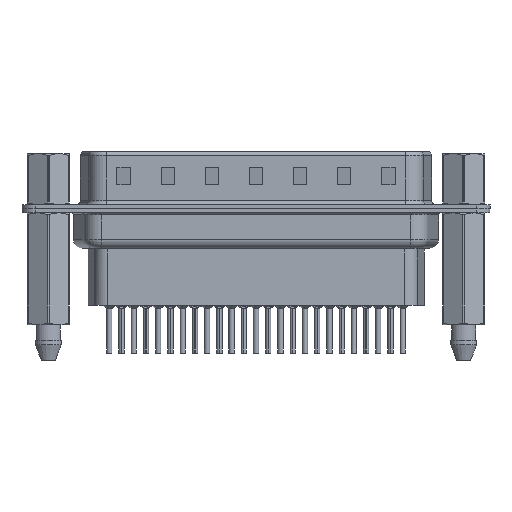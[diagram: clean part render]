
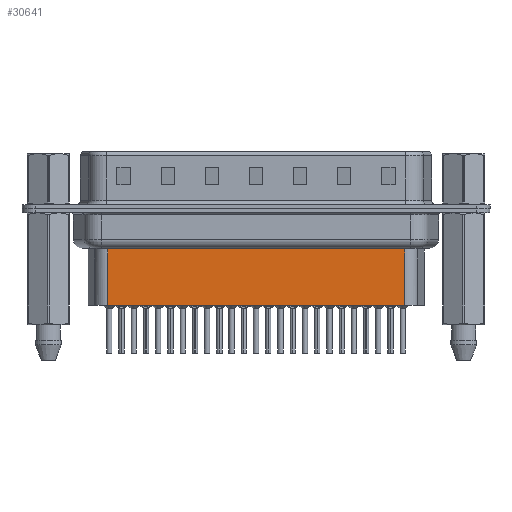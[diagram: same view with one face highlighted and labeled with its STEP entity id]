
A CAD part, front view. The second image highlights one B-rep face of the part: STEP entity #30641.
In plain terms, the highlighted planar face has unit normal (0, -1, 0).
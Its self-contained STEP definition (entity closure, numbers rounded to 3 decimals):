
#833 = AXIS2_PLACEMENT_3D ( 'NONE', #12504, #2280, #27858 ) ;
#1153 = ORIENTED_EDGE ( 'NONE', *, *, #26784, .F. ) ;
#1212 = EDGE_CURVE ( 'NONE', #7020, #14730, #2708, .T. ) ;
#2215 = EDGE_CURVE ( 'NONE', #14730, #2582, #17386, .T. ) ;
#2280 = DIRECTION ( 'NONE',  ( 0., -1., 0. ) ) ;
#2431 = PLANE ( 'NONE',  #833 ) ;
#2582 = VERTEX_POINT ( 'NONE', #17031 ) ;
#2708 = LINE ( 'NONE', #30763, #29126 ) ;
#4353 = VERTEX_POINT ( 'NONE', #31399 ) ;
#6843 = LINE ( 'NONE', #19389, #10309 ) ;
#7020 = VERTEX_POINT ( 'NONE', #22958 ) ;
#7847 = CARTESIAN_POINT ( 'NONE',  ( 40.344, -3.5, -3.1 ) ) ;
#10309 = VECTOR ( 'NONE', #21712, 1000. ) ;
#12504 = CARTESIAN_POINT ( 'NONE',  ( 6.706, -3.5, -3.1 ) ) ;
#13961 = ORIENTED_EDGE ( 'NONE', *, *, #1212, .T. ) ;
#14730 = VERTEX_POINT ( 'NONE', #31713 ) ;
#15062 = DIRECTION ( 'NONE',  ( 0., 0., -1. ) ) ;
#15328 = FACE_OUTER_BOUND ( 'NONE', #32353, .T. ) ;
#17031 = CARTESIAN_POINT ( 'NONE',  ( 6.706, -3.5, -10.95 ) ) ;
#17386 = LINE ( 'NONE', #27608, #23656 ) ;
#17885 = ORIENTED_EDGE ( 'NONE', *, *, #2215, .T. ) ;
#19389 = CARTESIAN_POINT ( 'NONE',  ( 6.706, -3.5, -10.95 ) ) ;
#20243 = LINE ( 'NONE', #7847, #20728 ) ;
#20728 = VECTOR ( 'NONE', #27650, 1000. ) ;
#21712 = DIRECTION ( 'NONE',  ( -1., 0., 0. ) ) ;
#22958 = CARTESIAN_POINT ( 'NONE',  ( 40.344, -3.5, -4.097 ) ) ;
#23656 = VECTOR ( 'NONE', #15062, 1000. ) ;
#24851 = ORIENTED_EDGE ( 'NONE', *, *, #28552, .F. ) ;
#26784 = EDGE_CURVE ( 'NONE', #7020, #4353, #20243, .T. ) ;
#27608 = CARTESIAN_POINT ( 'NONE',  ( 6.706, -3.5, -3.1 ) ) ;
#27650 = DIRECTION ( 'NONE',  ( 0., 0., -1. ) ) ;
#27858 = DIRECTION ( 'NONE',  ( 1., 0., 0. ) ) ;
#28552 = EDGE_CURVE ( 'NONE', #4353, #2582, #6843, .T. ) ;
#29126 = VECTOR ( 'NONE', #30427, 1000. ) ;
#30427 = DIRECTION ( 'NONE',  ( -1., 0., 0. ) ) ;
#30641 = ADVANCED_FACE ( 'NONE', ( #15328 ), #2431, .T. ) ;
#30763 = CARTESIAN_POINT ( 'NONE',  ( 6.459, -3.5, -4.097 ) ) ;
#31399 = CARTESIAN_POINT ( 'NONE',  ( 40.344, -3.5, -10.95 ) ) ;
#31713 = CARTESIAN_POINT ( 'NONE',  ( 6.706, -3.5, -4.097 ) ) ;
#32353 = EDGE_LOOP ( 'NONE', ( #1153, #13961, #17885, #24851 ) ) ;
